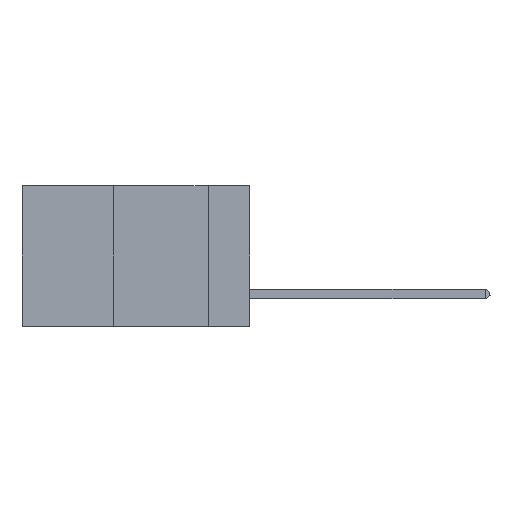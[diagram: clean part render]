
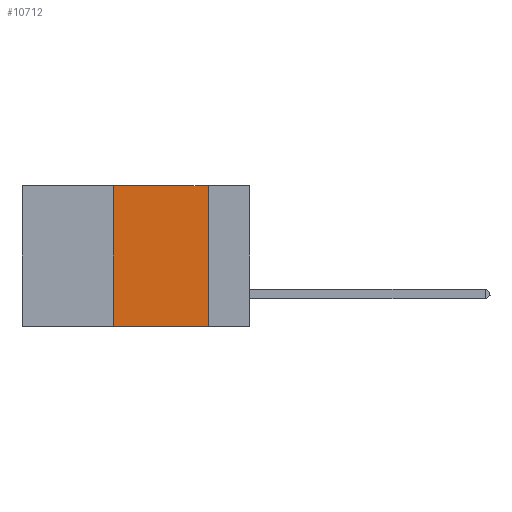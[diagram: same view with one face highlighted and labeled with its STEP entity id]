
A CAD part, left-side view. The second image highlights one B-rep face of the part: STEP entity #10712.
In plain terms, the highlighted planar face has unit normal (-1, 0, 0).
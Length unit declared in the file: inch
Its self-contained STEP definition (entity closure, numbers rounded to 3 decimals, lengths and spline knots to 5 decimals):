
#155 = EDGE_CURVE ( 'NONE', #2874, #1452, #7830, .T. ) ;
#1021 = VERTEX_POINT ( 'NONE', #4662 ) ;
#1235 = ORIENTED_EDGE ( 'NONE', *, *, #155, .F. ) ;
#1307 = CARTESIAN_POINT ( 'NONE',  ( 0., 0.36, 0. ) ) ;
#1452 = VERTEX_POINT ( 'NONE', #9209 ) ;
#1610 = VECTOR ( 'NONE', #3133, 39.37008 ) ;
#1649 = DIRECTION ( 'NONE',  ( 0., 0., -1. ) ) ;
#2073 = CARTESIAN_POINT ( 'NONE',  ( 0., 0.36, 0. ) ) ;
#2184 = ORIENTED_EDGE ( 'NONE', *, *, #5465, .F. ) ;
#2549 = CARTESIAN_POINT ( 'NONE',  ( 0., 0.11, -0.37 ) ) ;
#2556 = EDGE_CURVE ( 'NONE', #1452, #13144, #11127, .T. ) ;
#2675 = ORIENTED_EDGE ( 'NONE', *, *, #2556, .F. ) ;
#2874 = VERTEX_POINT ( 'NONE', #1307 ) ;
#2964 = VECTOR ( 'NONE', #11349, 39.37008 ) ;
#3133 = DIRECTION ( 'NONE',  ( 0., -1., 0. ) ) ;
#4332 = CARTESIAN_POINT ( 'NONE',  ( 0., 0.6, 0. ) ) ;
#4662 = CARTESIAN_POINT ( 'NONE',  ( 0., 0.36, -0.37 ) ) ;
#5406 = DIRECTION ( 'NONE',  ( 1., 0., 0. ) ) ;
#5465 = EDGE_CURVE ( 'NONE', #1021, #2874, #8176, .T. ) ;
#5773 = CARTESIAN_POINT ( 'NONE',  ( 0., 0.11, 0. ) ) ;
#6472 = DIRECTION ( 'NONE',  ( 0., 0., -1. ) ) ;
#6499 = AXIS2_PLACEMENT_3D ( 'NONE', #4332, #5406, #6472 ) ;
#6555 = EDGE_CURVE ( 'NONE', #1021, #13144, #13255, .T. ) ;
#7830 = LINE ( 'NONE', #11475, #2964 ) ;
#8176 = LINE ( 'NONE', #2073, #11209 ) ;
#8500 = PLANE ( 'NONE',  #6499 ) ;
#9209 = CARTESIAN_POINT ( 'NONE',  ( 0., 0.11, 0. ) ) ;
#9549 = DIRECTION ( 'NONE',  ( 0., 0., 1. ) ) ;
#9748 = ORIENTED_EDGE ( 'NONE', *, *, #6555, .T. ) ;
#9806 = EDGE_LOOP ( 'NONE', ( #2675, #1235, #2184, #9748 ) ) ;
#10712 = ADVANCED_FACE ( 'NONE', ( #12929 ), #8500, .F. ) ;
#11127 = LINE ( 'NONE', #5773, #11295 ) ;
#11209 = VECTOR ( 'NONE', #9549, 39.37008 ) ;
#11295 = VECTOR ( 'NONE', #1649, 39.37008 ) ;
#11349 = DIRECTION ( 'NONE',  ( 0., -1., 0. ) ) ;
#11475 = CARTESIAN_POINT ( 'NONE',  ( 0., 0.6, 0. ) ) ;
#12720 = CARTESIAN_POINT ( 'NONE',  ( 0., 0.6, -0.37 ) ) ;
#12929 = FACE_OUTER_BOUND ( 'NONE', #9806, .T. ) ;
#13144 = VERTEX_POINT ( 'NONE', #2549 ) ;
#13255 = LINE ( 'NONE', #12720, #1610 ) ;
